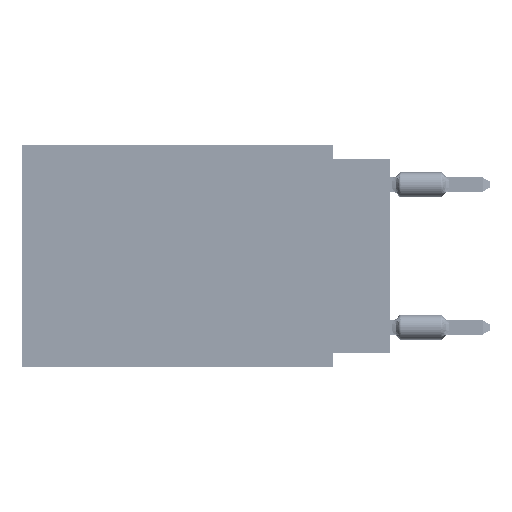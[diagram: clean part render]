
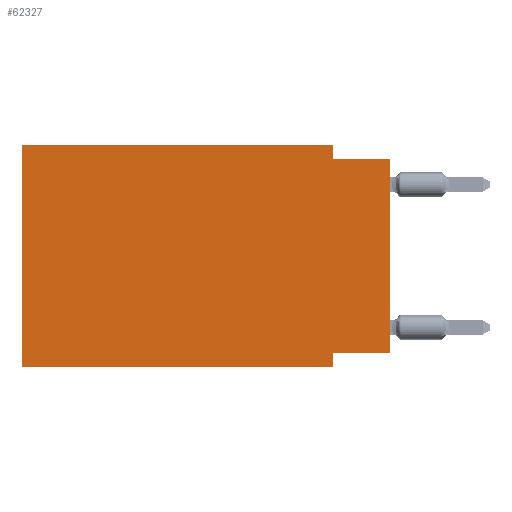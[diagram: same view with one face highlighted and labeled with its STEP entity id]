
A CAD part, left-side view. The second image highlights one B-rep face of the part: STEP entity #62327.
In plain terms, the highlighted planar face has unit normal (-1, 0, 0).
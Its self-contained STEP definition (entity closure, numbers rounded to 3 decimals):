
#877 = ORIENTED_EDGE ( 'NONE', *, *, #79368, .F. ) ;
#1091 = VECTOR ( 'NONE', #8502, 1000. ) ;
#1935 = DIRECTION ( 'NONE',  ( 1., 0., 0. ) ) ;
#6594 = VERTEX_POINT ( 'NONE', #57168 ) ;
#6887 = LINE ( 'NONE', #78712, #55926 ) ;
#8366 = EDGE_CURVE ( 'NONE', #68297, #30811, #50844, .T. ) ;
#8502 = DIRECTION ( 'NONE',  ( 0., -1., 0. ) ) ;
#9350 = CARTESIAN_POINT ( 'NONE',  ( 0., 16.383, 0. ) ) ;
#10670 = VERTEX_POINT ( 'NONE', #55767 ) ;
#12120 = LINE ( 'NONE', #84816, #30922 ) ;
#13732 = DIRECTION ( 'NONE',  ( 0., 0., -1. ) ) ;
#15428 = CARTESIAN_POINT ( 'NONE',  ( 0., 0., -0.635 ) ) ;
#16759 = ORIENTED_EDGE ( 'NONE', *, *, #68904, .T. ) ;
#17786 = DIRECTION ( 'NONE',  ( 0., 0., 1. ) ) ;
#19076 = DIRECTION ( 'NONE',  ( 0., 0., -1. ) ) ;
#21866 = ORIENTED_EDGE ( 'NONE', *, *, #40525, .F. ) ;
#22990 = CARTESIAN_POINT ( 'NONE',  ( 0., 16.383, -9.906 ) ) ;
#24205 = AXIS2_PLACEMENT_3D ( 'NONE', #74628, #1935, #13732 ) ;
#24503 = EDGE_CURVE ( 'NONE', #10670, #45705, #41190, .T. ) ;
#27633 = FACE_OUTER_BOUND ( 'NONE', #33995, .T. ) ;
#28360 = CARTESIAN_POINT ( 'NONE',  ( 0., 16.383, -9.906 ) ) ;
#29564 = LINE ( 'NONE', #77418, #75149 ) ;
#30811 = VERTEX_POINT ( 'NONE', #62860 ) ;
#30922 = VECTOR ( 'NONE', #38679, 1000. ) ;
#32919 = DIRECTION ( 'NONE',  ( 0., 0., 1. ) ) ;
#33995 = EDGE_LOOP ( 'NONE', ( #16759, #71119, #48254, #877, #21866, #64697, #73850, #55422 ) ) ;
#34894 = CARTESIAN_POINT ( 'NONE',  ( 0., 2.54, -9.271 ) ) ;
#36416 = VECTOR ( 'NONE', #32919, 1000. ) ;
#38679 = DIRECTION ( 'NONE',  ( 0., 1., 0. ) ) ;
#40525 = EDGE_CURVE ( 'NONE', #68297, #6594, #50063, .T. ) ;
#41190 = LINE ( 'NONE', #61188, #58627 ) ;
#45291 = EDGE_CURVE ( 'NONE', #55744, #67134, #12120, .T. ) ;
#45447 = EDGE_CURVE ( 'NONE', #67134, #30811, #6887, .T. ) ;
#45705 = VERTEX_POINT ( 'NONE', #51633 ) ;
#48187 = EDGE_CURVE ( 'NONE', #45705, #84018, #62392, .T. ) ;
#48254 = ORIENTED_EDGE ( 'NONE', *, *, #24503, .F. ) ;
#50063 = LINE ( 'NONE', #79052, #36416 ) ;
#50844 = LINE ( 'NONE', #22990, #52093 ) ;
#51633 = CARTESIAN_POINT ( 'NONE',  ( 0., 2.54, -0.635 ) ) ;
#52093 = VECTOR ( 'NONE', #76088, 1000. ) ;
#55422 = ORIENTED_EDGE ( 'NONE', *, *, #45291, .F. ) ;
#55744 = VERTEX_POINT ( 'NONE', #67507 ) ;
#55767 = CARTESIAN_POINT ( 'NONE',  ( 0., 2.54, 0. ) ) ;
#55926 = VECTOR ( 'NONE', #19076, 1000. ) ;
#57168 = CARTESIAN_POINT ( 'NONE',  ( 0., 16.383, 0. ) ) ;
#58627 = VECTOR ( 'NONE', #67737, 1000. ) ;
#61188 = CARTESIAN_POINT ( 'NONE',  ( 0., 2.54, 0. ) ) ;
#62327 = ADVANCED_FACE ( 'NONE', ( #27633 ), #73337, .F. ) ;
#62392 = LINE ( 'NONE', #15428, #72887 ) ;
#62860 = CARTESIAN_POINT ( 'NONE',  ( 0., 2.54, -9.906 ) ) ;
#64697 = ORIENTED_EDGE ( 'NONE', *, *, #8366, .T. ) ;
#67134 = VERTEX_POINT ( 'NONE', #34894 ) ;
#67507 = CARTESIAN_POINT ( 'NONE',  ( 0., 0., -9.271 ) ) ;
#67737 = DIRECTION ( 'NONE',  ( 0., 0., -1. ) ) ;
#68297 = VERTEX_POINT ( 'NONE', #28360 ) ;
#68522 = DIRECTION ( 'NONE',  ( 0., -1., 0. ) ) ;
#68904 = EDGE_CURVE ( 'NONE', #55744, #84018, #29564, .T. ) ;
#68973 = LINE ( 'NONE', #9350, #1091 ) ;
#71119 = ORIENTED_EDGE ( 'NONE', *, *, #48187, .F. ) ;
#72887 = VECTOR ( 'NONE', #68522, 1000. ) ;
#73337 = PLANE ( 'NONE',  #24205 ) ;
#73850 = ORIENTED_EDGE ( 'NONE', *, *, #45447, .F. ) ;
#74628 = CARTESIAN_POINT ( 'NONE',  ( 0., 16.383, 0. ) ) ;
#75149 = VECTOR ( 'NONE', #17786, 1000. ) ;
#76088 = DIRECTION ( 'NONE',  ( 0., -1., 0. ) ) ;
#76767 = CARTESIAN_POINT ( 'NONE',  ( 0., 0., -0.635 ) ) ;
#77418 = CARTESIAN_POINT ( 'NONE',  ( 0., 0., 0. ) ) ;
#78712 = CARTESIAN_POINT ( 'NONE',  ( 0., 2.54, -9.906 ) ) ;
#79052 = CARTESIAN_POINT ( 'NONE',  ( 0., 16.383, 0. ) ) ;
#79368 = EDGE_CURVE ( 'NONE', #6594, #10670, #68973, .T. ) ;
#84018 = VERTEX_POINT ( 'NONE', #76767 ) ;
#84816 = CARTESIAN_POINT ( 'NONE',  ( 0., 0., -9.271 ) ) ;
